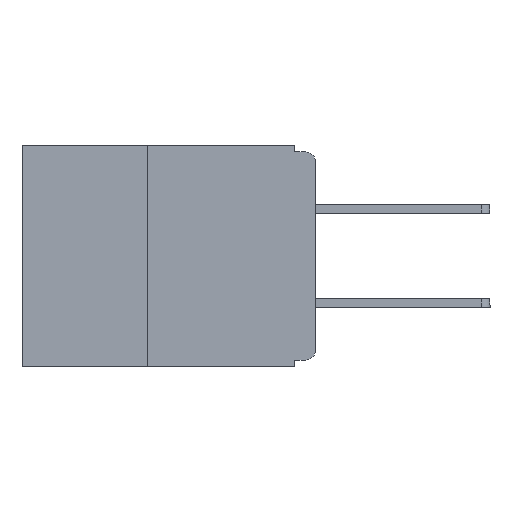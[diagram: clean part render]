
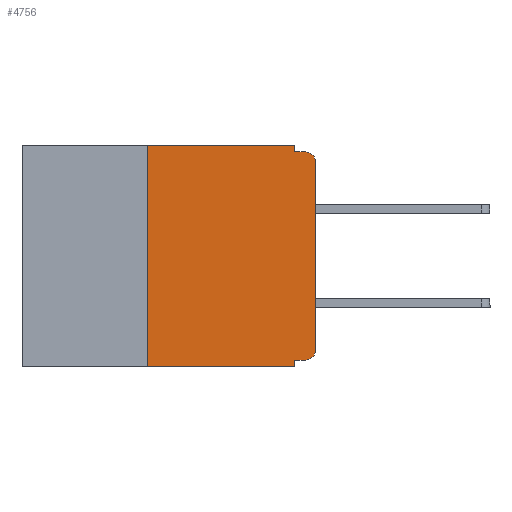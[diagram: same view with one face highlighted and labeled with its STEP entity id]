
A CAD part, left-side view. The second image highlights one B-rep face of the part: STEP entity #4756.
In plain terms, the highlighted planar face has unit normal (-1, 0, 0).
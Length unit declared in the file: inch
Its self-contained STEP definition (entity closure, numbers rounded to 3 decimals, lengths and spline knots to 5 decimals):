
#225 = VECTOR ( 'NONE', #5723, 39.37008 ) ;
#382 = ORIENTED_EDGE ( 'NONE', *, *, #13317, .F. ) ;
#513 = VECTOR ( 'NONE', #21467, 39.37008 ) ;
#514 = CARTESIAN_POINT ( 'NONE',  ( 0., 0.015, -0.32 ) ) ;
#883 = CARTESIAN_POINT ( 'NONE',  ( 0., 0.25, 0. ) ) ;
#1069 = VECTOR ( 'NONE', #3280, 39.37008 ) ;
#1298 = ORIENTED_EDGE ( 'NONE', *, *, #7087, .F. ) ;
#1443 = LINE ( 'NONE', #21280, #225 ) ;
#1871 = AXIS2_PLACEMENT_3D ( 'NONE', #18783, #20267, #9822 ) ;
#2490 = CIRCLE ( 'NONE', #17046, 0.015 ) ;
#2793 = EDGE_CURVE ( 'NONE', #7560, #17393, #1443, .T. ) ;
#3258 = DIRECTION ( 'NONE',  ( 0., 1., 0. ) ) ;
#3280 = DIRECTION ( 'NONE',  ( 0., -1., 0. ) ) ;
#3415 = PLANE ( 'NONE',  #1871 ) ;
#3941 = CARTESIAN_POINT ( 'NONE',  ( 0., 0.031, -0.33 ) ) ;
#4500 = VERTEX_POINT ( 'NONE', #11466 ) ;
#4756 = ADVANCED_FACE ( 'NONE', ( #9450 ), #3415, .F. ) ;
#4786 = CARTESIAN_POINT ( 'NONE',  ( 0., 0., -0.025 ) ) ;
#5020 = LINE ( 'NONE', #10966, #14672 ) ;
#5071 = VECTOR ( 'NONE', #10101, 39.37008 ) ;
#5535 = CARTESIAN_POINT ( 'NONE',  ( 0., 0.437, 0. ) ) ;
#5723 = DIRECTION ( 'NONE',  ( 0., 0., 1. ) ) ;
#5895 = EDGE_CURVE ( 'NONE', #20583, #14209, #14217, .T. ) ;
#6253 = EDGE_CURVE ( 'NONE', #14209, #4500, #21086, .T. ) ;
#6896 = VECTOR ( 'NONE', #16495, 39.37008 ) ;
#7087 = EDGE_CURVE ( 'NONE', #12580, #20583, #12027, .T. ) ;
#7465 = CARTESIAN_POINT ( 'NONE',  ( 0., 0., -0.305 ) ) ;
#7560 = VERTEX_POINT ( 'NONE', #7465 ) ;
#7941 = EDGE_CURVE ( 'NONE', #9498, #22699, #12594, .T. ) ;
#8048 = ORIENTED_EDGE ( 'NONE', *, *, #14677, .T. ) ;
#8653 = VERTEX_POINT ( 'NONE', #13586 ) ;
#8874 = VECTOR ( 'NONE', #9836, 39.37008 ) ;
#9341 = DIRECTION ( 'NONE',  ( -1., 0., 0. ) ) ;
#9450 = FACE_OUTER_BOUND ( 'NONE', #16051, .T. ) ;
#9498 = VERTEX_POINT ( 'NONE', #15192 ) ;
#9822 = DIRECTION ( 'NONE',  ( 0., 0., -1. ) ) ;
#9836 = DIRECTION ( 'NONE',  ( 0., -1., 0. ) ) ;
#10101 = DIRECTION ( 'NONE',  ( 0., 0., 1. ) ) ;
#10197 = LINE ( 'NONE', #17788, #5071 ) ;
#10625 = DIRECTION ( 'NONE',  ( -1., 0., 0. ) ) ;
#10966 = CARTESIAN_POINT ( 'NONE',  ( 0., 0., -0.32 ) ) ;
#11466 = CARTESIAN_POINT ( 'NONE',  ( 0., 0.015, -0.01 ) ) ;
#12027 = LINE ( 'NONE', #5535, #1069 ) ;
#12144 = CARTESIAN_POINT ( 'NONE',  ( 0., 0.031, -0.33 ) ) ;
#12247 = ORIENTED_EDGE ( 'NONE', *, *, #22371, .T. ) ;
#12396 = EDGE_CURVE ( 'NONE', #8653, #12580, #10197, .T. ) ;
#12462 = CIRCLE ( 'NONE', #13366, 0.015 ) ;
#12580 = VERTEX_POINT ( 'NONE', #883 ) ;
#12594 = LINE ( 'NONE', #12144, #6896 ) ;
#12864 = ORIENTED_EDGE ( 'NONE', *, *, #5895, .F. ) ;
#13317 = EDGE_CURVE ( 'NONE', #18033, #9498, #5020, .T. ) ;
#13366 = AXIS2_PLACEMENT_3D ( 'NONE', #22161, #10625, #24032 ) ;
#13586 = CARTESIAN_POINT ( 'NONE',  ( 0., 0.25, -0.33 ) ) ;
#13622 = VECTOR ( 'NONE', #16629, 39.37008 ) ;
#14209 = VERTEX_POINT ( 'NONE', #23265 ) ;
#14217 = LINE ( 'NONE', #16745, #13622 ) ;
#14672 = VECTOR ( 'NONE', #3258, 39.37008 ) ;
#14677 = EDGE_CURVE ( 'NONE', #8653, #22699, #22996, .T. ) ;
#15192 = CARTESIAN_POINT ( 'NONE',  ( 0., 0.031, -0.32 ) ) ;
#16051 = EDGE_LOOP ( 'NONE', ( #22508, #21592, #18007, #12864, #1298, #21266, #8048, #22175, #382, #12247 ) ) ;
#16495 = DIRECTION ( 'NONE',  ( 0., 0., -1. ) ) ;
#16629 = DIRECTION ( 'NONE',  ( 0., 0., -1. ) ) ;
#16745 = CARTESIAN_POINT ( 'NONE',  ( 0., 0.031, 0. ) ) ;
#17046 = AXIS2_PLACEMENT_3D ( 'NONE', #20839, #9341, #22772 ) ;
#17393 = VERTEX_POINT ( 'NONE', #4786 ) ;
#17574 = EDGE_CURVE ( 'NONE', #17393, #4500, #2490, .T. ) ;
#17788 = CARTESIAN_POINT ( 'NONE',  ( 0., 0.25, -0.33 ) ) ;
#18007 = ORIENTED_EDGE ( 'NONE', *, *, #6253, .F. ) ;
#18033 = VERTEX_POINT ( 'NONE', #514 ) ;
#18783 = CARTESIAN_POINT ( 'NONE',  ( 0., 0.437, 0. ) ) ;
#20267 = DIRECTION ( 'NONE',  ( 1., 0., 0. ) ) ;
#20583 = VERTEX_POINT ( 'NONE', #22221 ) ;
#20839 = CARTESIAN_POINT ( 'NONE',  ( 0., 0.015, -0.025 ) ) ;
#21086 = LINE ( 'NONE', #21383, #513 ) ;
#21266 = ORIENTED_EDGE ( 'NONE', *, *, #12396, .F. ) ;
#21280 = CARTESIAN_POINT ( 'NONE',  ( 0., 0., 0. ) ) ;
#21339 = CARTESIAN_POINT ( 'NONE',  ( 0., 0.437, -0.33 ) ) ;
#21383 = CARTESIAN_POINT ( 'NONE',  ( 0., 0., -0.01 ) ) ;
#21467 = DIRECTION ( 'NONE',  ( 0., -1., 0. ) ) ;
#21592 = ORIENTED_EDGE ( 'NONE', *, *, #17574, .T. ) ;
#22161 = CARTESIAN_POINT ( 'NONE',  ( 0., 0.015, -0.305 ) ) ;
#22175 = ORIENTED_EDGE ( 'NONE', *, *, #7941, .F. ) ;
#22221 = CARTESIAN_POINT ( 'NONE',  ( 0., 0.031, 0. ) ) ;
#22371 = EDGE_CURVE ( 'NONE', #18033, #7560, #12462, .T. ) ;
#22508 = ORIENTED_EDGE ( 'NONE', *, *, #2793, .T. ) ;
#22699 = VERTEX_POINT ( 'NONE', #3941 ) ;
#22772 = DIRECTION ( 'NONE',  ( 0., 0., -1. ) ) ;
#22996 = LINE ( 'NONE', #21339, #8874 ) ;
#23265 = CARTESIAN_POINT ( 'NONE',  ( 0., 0.031, -0.01 ) ) ;
#24032 = DIRECTION ( 'NONE',  ( 0., 0., -1. ) ) ;
